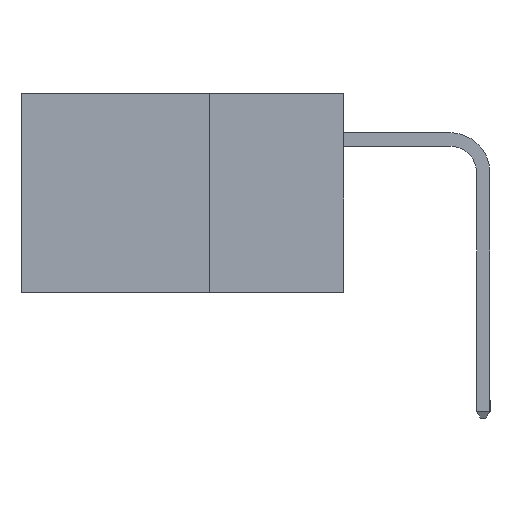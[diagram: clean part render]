
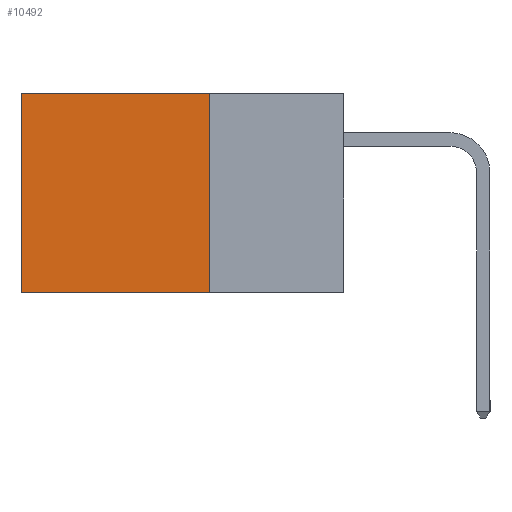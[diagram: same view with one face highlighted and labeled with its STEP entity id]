
A CAD part, left-side view. The second image highlights one B-rep face of the part: STEP entity #10492.
In plain terms, the highlighted planar face has unit normal (-1, 0, 0).
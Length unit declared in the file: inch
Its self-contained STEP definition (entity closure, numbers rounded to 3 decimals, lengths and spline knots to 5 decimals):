
#298 = CARTESIAN_POINT ( 'NONE',  ( 0.2615, 0.6, -0.37 ) ) ;
#353 = VERTEX_POINT ( 'NONE', #6068 ) ;
#674 = CARTESIAN_POINT ( 'NONE',  ( 0.2615, 0.25, -0.37 ) ) ;
#1311 = ORIENTED_EDGE ( 'NONE', *, *, #8590, .T. ) ;
#1341 = ORIENTED_EDGE ( 'NONE', *, *, #6239, .T. ) ;
#1743 = ORIENTED_EDGE ( 'NONE', *, *, #7126, .F. ) ;
#2817 = PLANE ( 'NONE',  #8247 ) ;
#2834 = LINE ( 'NONE', #674, #7179 ) ;
#3617 = FACE_OUTER_BOUND ( 'NONE', #9266, .T. ) ;
#3719 = DIRECTION ( 'NONE',  ( 1., 0., 0. ) ) ;
#4311 = LINE ( 'NONE', #9539, #4872 ) ;
#4508 = DIRECTION ( 'NONE',  ( 0., 1., 0. ) ) ;
#4554 = VERTEX_POINT ( 'NONE', #10759 ) ;
#4872 = VECTOR ( 'NONE', #4508, 39.37008 ) ;
#5184 = CARTESIAN_POINT ( 'NONE',  ( 0.2615, 0.25, 0. ) ) ;
#5391 = VERTEX_POINT ( 'NONE', #5184 ) ;
#5615 = DIRECTION ( 'NONE',  ( 0., 0., -1. ) ) ;
#6068 = CARTESIAN_POINT ( 'NONE',  ( 0.2615, 0.6, 0. ) ) ;
#6239 = EDGE_CURVE ( 'NONE', #353, #7449, #7650, .T. ) ;
#6354 = VECTOR ( 'NONE', #9133, 39.37008 ) ;
#6627 = LINE ( 'NONE', #8303, #6354 ) ;
#6777 = CARTESIAN_POINT ( 'NONE',  ( 0.2615, 0.6, -0.37 ) ) ;
#7126 = EDGE_CURVE ( 'NONE', #4554, #7449, #4311, .T. ) ;
#7179 = VECTOR ( 'NONE', #10882, 39.37008 ) ;
#7449 = VERTEX_POINT ( 'NONE', #6777 ) ;
#7650 = LINE ( 'NONE', #298, #9597 ) ;
#8098 = EDGE_CURVE ( 'NONE', #5391, #4554, #2834, .T. ) ;
#8247 = AXIS2_PLACEMENT_3D ( 'NONE', #8825, #3719, #9629 ) ;
#8303 = CARTESIAN_POINT ( 'NONE',  ( 0.2615, 0.25, 0. ) ) ;
#8428 = ORIENTED_EDGE ( 'NONE', *, *, #8098, .F. ) ;
#8590 = EDGE_CURVE ( 'NONE', #5391, #353, #6627, .T. ) ;
#8825 = CARTESIAN_POINT ( 'NONE',  ( 0.2615, 0.25, -0.37 ) ) ;
#9133 = DIRECTION ( 'NONE',  ( 0., 1., 0. ) ) ;
#9266 = EDGE_LOOP ( 'NONE', ( #1341, #1743, #8428, #1311 ) ) ;
#9539 = CARTESIAN_POINT ( 'NONE',  ( 0.2615, 0.25, -0.37 ) ) ;
#9597 = VECTOR ( 'NONE', #5615, 39.37008 ) ;
#9629 = DIRECTION ( 'NONE',  ( 0., 0., -1. ) ) ;
#10492 = ADVANCED_FACE ( 'NONE', ( #3617 ), #2817, .F. ) ;
#10759 = CARTESIAN_POINT ( 'NONE',  ( 0.2615, 0.25, -0.37 ) ) ;
#10882 = DIRECTION ( 'NONE',  ( 0., 0., -1. ) ) ;
